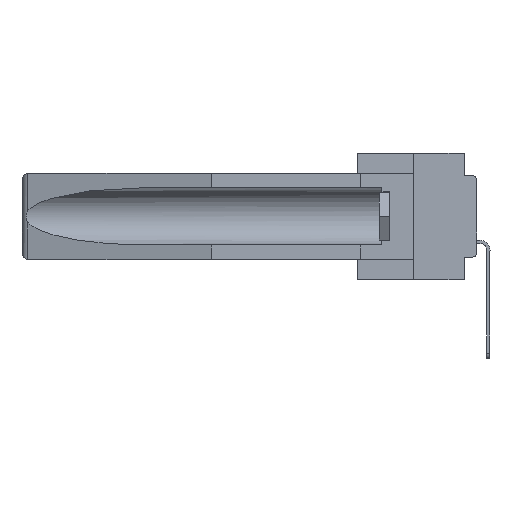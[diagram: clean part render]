
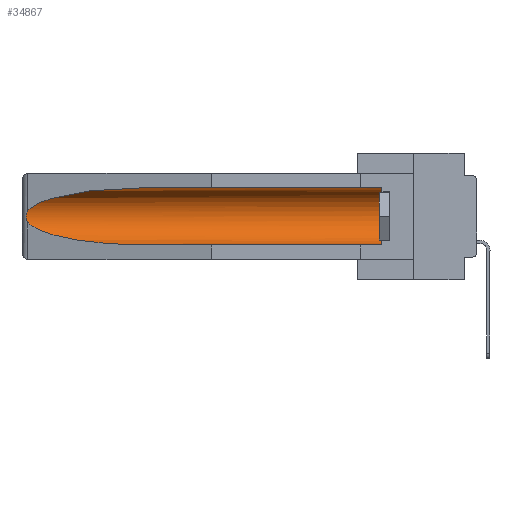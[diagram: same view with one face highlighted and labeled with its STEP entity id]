
A CAD part, left-side view. The second image highlights one B-rep face of the part: STEP entity #34867.
In plain terms, the highlighted cylindrical face has radius 2.857 mm (diameter 5.715 mm), a partial arc.
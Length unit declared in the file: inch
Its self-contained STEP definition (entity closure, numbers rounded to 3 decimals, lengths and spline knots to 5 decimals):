
#1167 = CARTESIAN_POINT ( 'NONE',  ( 0.155, -0.30754, -0.1715 ) ) ;
#1485 = ORIENTED_EDGE ( 'NONE', *, *, #14787, .T. ) ;
#1708 = CARTESIAN_POINT ( 'NONE',  ( 0.155, 0.126, -0.284 ) ) ;
#3036 = CARTESIAN_POINT ( 'NONE',  ( 0.26537, 1.52718, -0.19328 ) ) ;
#3232 = CARTESIAN_POINT ( 'NONE',  ( 0.155, 1.07973, -0.059 ) ) ;
#3330 = EDGE_CURVE ( 'NONE', #21138, #24465, #18163, .T. ) ;
#4045 = EDGE_CURVE ( 'NONE', #27644, #25650, #5002, .T. ) ;
#4120 = CARTESIAN_POINT ( 'NONE',  ( 0.155, 1.07973, -0.059 ) ) ;
#4242 = CARTESIAN_POINT ( 'NONE',  ( 0.26597, 1.52961, -0.15275 ) ) ;
#4714 = CARTESIAN_POINT ( 'NONE',  ( 0.26655, 1.53094, -0.18657 ) ) ;
#5002 = B_SPLINE_CURVE_WITH_KNOTS ( 'NONE', 3,
 ( #17945, #4242, #6951, #26211, #33928, #18081, #31472, #4714, #33795, #18201 ),
 .UNSPECIFIED., .F., .F.,
 ( 4, 2, 2, 2, 4 ),
 ( 0., 0.00029, 0.00058, 0.00087, 0.00117 ),
 .UNSPECIFIED. ) ;
#5395 = AXIS2_PLACEMENT_3D ( 'NONE', #1167, #9166, #17821 ) ;
#6881 = DIRECTION ( 'NONE',  ( 0., 1., 0. ) ) ;
#6951 = CARTESIAN_POINT ( 'NONE',  ( 0.26654, 1.53092, -0.15636 ) ) ;
#7600 =( BOUNDED_CURVE ( )  B_SPLINE_CURVE ( 3, ( #32139, #7871, #18746, #13497 ),
 .UNSPECIFIED., .F., .F. ) 
 B_SPLINE_CURVE_WITH_KNOTS ( ( 4, 4 ),
 ( 0.1948, 1.5708 ),
 .UNSPECIFIED. ) 
 CURVE ( )  GEOMETRIC_REPRESENTATION_ITEM ( )  RATIONAL_B_SPLINE_CURVE ( ( 1., 0.848, 0.848, 1. ) ) 
 REPRESENTATION_ITEM ( '' )  );
#7700 = CARTESIAN_POINT ( 'NONE',  ( 0.155, 1.07973, -0.284 ) ) ;
#7871 = CARTESIAN_POINT ( 'NONE',  ( 0.25451, 1.48313, -0.24835 ) ) ;
#8679 = CARTESIAN_POINT ( 'NONE',  ( 0.155, 0.126, -0.059 ) ) ;
#9166 = DIRECTION ( 'NONE',  ( 0., 1., 0. ) ) ;
#10205 = CARTESIAN_POINT ( 'NONE',  ( 0.26537, 1.52718, -0.14972 ) ) ;
#10904 = VECTOR ( 'NONE', #6881, 39.37008 ) ;
#12220 = CARTESIAN_POINT ( 'NONE',  ( 0.155, 0.126, -0.1715 ) ) ;
#13356 = ORIENTED_EDGE ( 'NONE', *, *, #16706, .T. ) ;
#13497 = CARTESIAN_POINT ( 'NONE',  ( 0.155, 1.07973, -0.284 ) ) ;
#13732 = ORIENTED_EDGE ( 'NONE', *, *, #3330, .T. ) ;
#14766 = VECTOR ( 'NONE', #14893, 39.37008 ) ;
#14787 = EDGE_CURVE ( 'NONE', #24465, #27644, #23854, .T. ) ;
#14893 = DIRECTION ( 'NONE',  ( 0., 1., 0. ) ) ;
#16706 = EDGE_CURVE ( 'NONE', #26554, #21138, #25302, .T. ) ;
#17326 = CARTESIAN_POINT ( 'NONE',  ( 0.26537, 1.52718, -0.14972 ) ) ;
#17821 = DIRECTION ( 'NONE',  ( 0., 0., 1. ) ) ;
#17945 = CARTESIAN_POINT ( 'NONE',  ( 0.26537, 1.52718, -0.14972 ) ) ;
#18081 = CARTESIAN_POINT ( 'NONE',  ( 0.2675, 1.53308, -0.17534 ) ) ;
#18163 = LINE ( 'NONE', #22477, #10904 ) ;
#18201 = CARTESIAN_POINT ( 'NONE',  ( 0.26537, 1.52718, -0.19328 ) ) ;
#18746 = CARTESIAN_POINT ( 'NONE',  ( 0.21114, 1.30732, -0.284 ) ) ;
#20252 = DIRECTION ( 'NONE',  ( 0., -1., 0. ) ) ;
#20332 = VERTEX_POINT ( 'NONE', #7700 ) ;
#20444 = CARTESIAN_POINT ( 'NONE',  ( 0.155, -0.30754, -0.284 ) ) ;
#21138 = VERTEX_POINT ( 'NONE', #8679 ) ;
#21897 = ORIENTED_EDGE ( 'NONE', *, *, #24384, .T. ) ;
#22477 = CARTESIAN_POINT ( 'NONE',  ( 0.155, -0.30754, -0.059 ) ) ;
#23854 =( BOUNDED_CURVE ( )  B_SPLINE_CURVE ( 3, ( #4120, #25488, #28432, #17326 ),
 .UNSPECIFIED., .F., .F. ) 
 B_SPLINE_CURVE_WITH_KNOTS ( ( 4, 4 ),
 ( 4.71239, 6.08839 ),
 .UNSPECIFIED. ) 
 CURVE ( )  GEOMETRIC_REPRESENTATION_ITEM ( )  RATIONAL_B_SPLINE_CURVE ( ( 1., 0.848, 0.848, 1. ) ) 
 REPRESENTATION_ITEM ( '' )  );
#24369 = ORIENTED_EDGE ( 'NONE', *, *, #30305, .F. ) ;
#24384 = EDGE_CURVE ( 'NONE', #25650, #20332, #7600, .T. ) ;
#24465 = VERTEX_POINT ( 'NONE', #3232 ) ;
#25225 = DIRECTION ( 'NONE',  ( 0., 0., 1. ) ) ;
#25302 = CIRCLE ( 'NONE', #29170, 0.1125 ) ;
#25488 = CARTESIAN_POINT ( 'NONE',  ( 0.21114, 1.30732, -0.059 ) ) ;
#25650 = VERTEX_POINT ( 'NONE', #3036 ) ;
#26211 = CARTESIAN_POINT ( 'NONE',  ( 0.2673, 1.5327, -0.16383 ) ) ;
#26554 = VERTEX_POINT ( 'NONE', #1708 ) ;
#27040 = LINE ( 'NONE', #20444, #14766 ) ;
#27644 = VERTEX_POINT ( 'NONE', #10205 ) ;
#28432 = CARTESIAN_POINT ( 'NONE',  ( 0.25451, 1.48313, -0.09465 ) ) ;
#29170 = AXIS2_PLACEMENT_3D ( 'NONE', #12220, #20252, #25225 ) ;
#29683 = CYLINDRICAL_SURFACE ( 'NONE', #5395, 0.1125 ) ;
#30305 = EDGE_CURVE ( 'NONE', #26554, #20332, #27040, .T. ) ;
#30675 = EDGE_LOOP ( 'NONE', ( #1485, #34430, #21897, #24369, #13356, #13732 ) ) ;
#31472 = CARTESIAN_POINT ( 'NONE',  ( 0.2673, 1.53269, -0.17917 ) ) ;
#32139 = CARTESIAN_POINT ( 'NONE',  ( 0.26537, 1.52718, -0.19328 ) ) ;
#33795 = CARTESIAN_POINT ( 'NONE',  ( 0.26597, 1.5296, -0.19026 ) ) ;
#33889 = FACE_OUTER_BOUND ( 'NONE', #30675, .T. ) ;
#33928 = CARTESIAN_POINT ( 'NONE',  ( 0.2675, 1.53308, -0.16763 ) ) ;
#34430 = ORIENTED_EDGE ( 'NONE', *, *, #4045, .T. ) ;
#34867 = ADVANCED_FACE ( 'NONE', ( #33889 ), #29683, .F. ) ;
